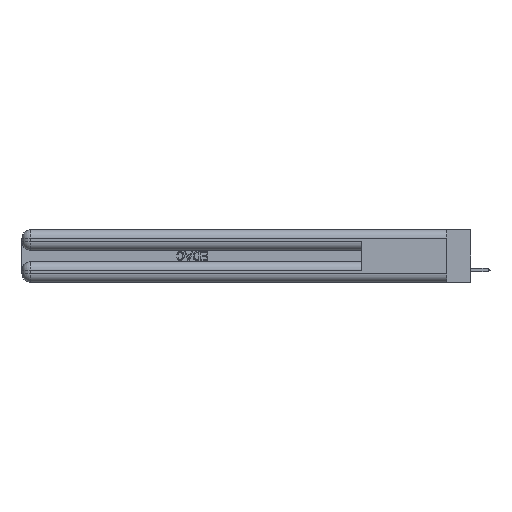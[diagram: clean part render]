
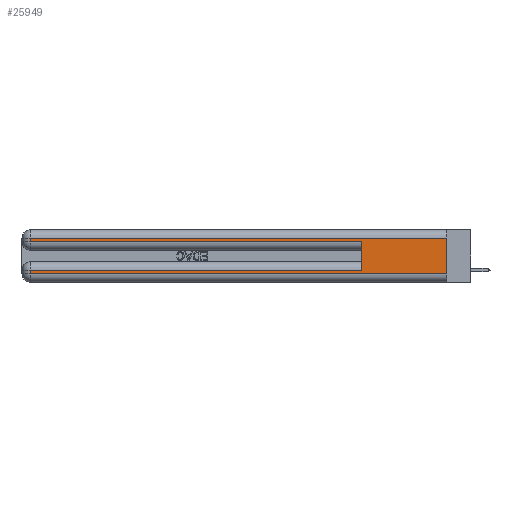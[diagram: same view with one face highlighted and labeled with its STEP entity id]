
A CAD part, left-side view. The second image highlights one B-rep face of the part: STEP entity #25949.
In plain terms, the highlighted planar face has unit normal (-1, 0, 0).
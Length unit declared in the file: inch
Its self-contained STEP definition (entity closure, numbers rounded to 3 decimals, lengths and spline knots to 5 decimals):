
#247 = CARTESIAN_POINT ( 'NONE',  ( 0., 0., 0.37 ) ) ;
#284 = CARTESIAN_POINT ( 'NONE',  ( 0., 0.6, 0.145 ) ) ;
#358 = EDGE_CURVE ( 'NONE', #15096, #21824, #19741, .T. ) ;
#1117 = LINE ( 'NONE', #5309, #30140 ) ;
#1136 = EDGE_CURVE ( 'NONE', #15096, #8211, #34162, .T. ) ;
#2267 = VERTEX_POINT ( 'NONE', #35709 ) ;
#2771 = VECTOR ( 'NONE', #23647, 39.37008 ) ;
#2908 = DIRECTION ( 'NONE',  ( 0., 0., -1. ) ) ;
#2916 = EDGE_CURVE ( 'NONE', #29318, #4065, #26981, .T. ) ;
#3358 = ORIENTED_EDGE ( 'NONE', *, *, #358, .F. ) ;
#4065 = VERTEX_POINT ( 'NONE', #25285 ) ;
#4449 = ORIENTED_EDGE ( 'NONE', *, *, #1136, .T. ) ;
#4608 = VERTEX_POINT ( 'NONE', #13046 ) ;
#4953 = VECTOR ( 'NONE', #6447, 39.37008 ) ;
#5114 = ORIENTED_EDGE ( 'NONE', *, *, #6829, .T. ) ;
#5269 = DIRECTION ( 'NONE',  ( 0., 0., 1. ) ) ;
#5309 = CARTESIAN_POINT ( 'NONE',  ( 0., 2.94, 0.37 ) ) ;
#6441 = VECTOR ( 'NONE', #20477, 39.37008 ) ;
#6447 = DIRECTION ( 'NONE',  ( 0., -1., 0. ) ) ;
#6829 = EDGE_CURVE ( 'NONE', #28622, #4608, #10462, .T. ) ;
#7300 = EDGE_LOOP ( 'NONE', ( #24659, #29412, #5114, #19661, #3358, #4449, #14967, #31991 ) ) ;
#7799 = DIRECTION ( 'NONE',  ( 0., 1., 0. ) ) ;
#8211 = VERTEX_POINT ( 'NONE', #13967 ) ;
#8490 = LINE ( 'NONE', #33146, #8911 ) ;
#8567 = DIRECTION ( 'NONE',  ( 0., 0., -1. ) ) ;
#8911 = VECTOR ( 'NONE', #25458, 39.37008 ) ;
#10043 = EDGE_CURVE ( 'NONE', #2267, #4065, #19894, .T. ) ;
#10462 = LINE ( 'NONE', #14652, #22329 ) ;
#11118 = LINE ( 'NONE', #15968, #26035 ) ;
#13046 = CARTESIAN_POINT ( 'NONE',  ( 0., 2.94, 0.285 ) ) ;
#13967 = CARTESIAN_POINT ( 'NONE',  ( 0., 2.94, 0.085 ) ) ;
#14652 = CARTESIAN_POINT ( 'NONE',  ( 0., 2.94, 0.37 ) ) ;
#14967 = ORIENTED_EDGE ( 'NONE', *, *, #15367, .T. ) ;
#15096 = VERTEX_POINT ( 'NONE', #16032 ) ;
#15367 = EDGE_CURVE ( 'NONE', #8211, #2267, #1117, .T. ) ;
#15968 = CARTESIAN_POINT ( 'NONE',  ( 0., 0., 0.31 ) ) ;
#16032 = CARTESIAN_POINT ( 'NONE',  ( 0., 0.6, 0.085 ) ) ;
#16240 = EDGE_CURVE ( 'NONE', #4608, #21824, #8490, .T. ) ;
#17095 = VECTOR ( 'NONE', #5269, 39.37008 ) ;
#17789 = FACE_OUTER_BOUND ( 'NONE', #7300, .T. ) ;
#19661 = ORIENTED_EDGE ( 'NONE', *, *, #16240, .T. ) ;
#19741 = LINE ( 'NONE', #284, #17095 ) ;
#19894 = LINE ( 'NONE', #28717, #4953 ) ;
#20108 = EDGE_CURVE ( 'NONE', #29318, #28622, #11118, .T. ) ;
#20219 = CARTESIAN_POINT ( 'NONE',  ( 0., 0., 0.085 ) ) ;
#20477 = DIRECTION ( 'NONE',  ( 0., 1., 0. ) ) ;
#20903 = CARTESIAN_POINT ( 'NONE',  ( 0., 0., 0.37 ) ) ;
#21824 = VERTEX_POINT ( 'NONE', #23062 ) ;
#22329 = VECTOR ( 'NONE', #8567, 39.37008 ) ;
#22406 = DIRECTION ( 'NONE',  ( 0., 0., -1. ) ) ;
#22643 = AXIS2_PLACEMENT_3D ( 'NONE', #247, #25396, #2908 ) ;
#23062 = CARTESIAN_POINT ( 'NONE',  ( 0., 0.6, 0.285 ) ) ;
#23097 = PLANE ( 'NONE',  #22643 ) ;
#23647 = DIRECTION ( 'NONE',  ( 0., 0., -1. ) ) ;
#24220 = CARTESIAN_POINT ( 'NONE',  ( 0., 2.94, 0.31 ) ) ;
#24408 = CARTESIAN_POINT ( 'NONE',  ( 0., 0., 0.31 ) ) ;
#24659 = ORIENTED_EDGE ( 'NONE', *, *, #2916, .F. ) ;
#25285 = CARTESIAN_POINT ( 'NONE',  ( 0., 0., 0.06 ) ) ;
#25396 = DIRECTION ( 'NONE',  ( 1., 0., 0. ) ) ;
#25458 = DIRECTION ( 'NONE',  ( 0., -1., 0. ) ) ;
#25949 = ADVANCED_FACE ( 'NONE', ( #17789 ), #23097, .F. ) ;
#26035 = VECTOR ( 'NONE', #7799, 39.37008 ) ;
#26981 = LINE ( 'NONE', #20903, #2771 ) ;
#28622 = VERTEX_POINT ( 'NONE', #24220 ) ;
#28717 = CARTESIAN_POINT ( 'NONE',  ( 0., 0., 0.06 ) ) ;
#29318 = VERTEX_POINT ( 'NONE', #24408 ) ;
#29412 = ORIENTED_EDGE ( 'NONE', *, *, #20108, .T. ) ;
#30140 = VECTOR ( 'NONE', #22406, 39.37008 ) ;
#31991 = ORIENTED_EDGE ( 'NONE', *, *, #10043, .T. ) ;
#33146 = CARTESIAN_POINT ( 'NONE',  ( 0., 0., 0.285 ) ) ;
#34162 = LINE ( 'NONE', #20219, #6441 ) ;
#35709 = CARTESIAN_POINT ( 'NONE',  ( 0., 2.94, 0.06 ) ) ;
